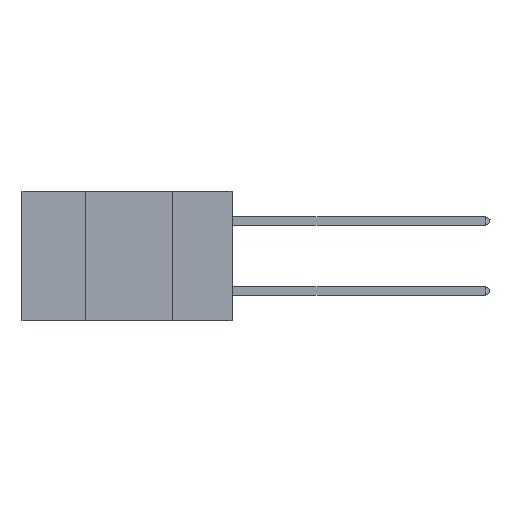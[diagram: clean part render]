
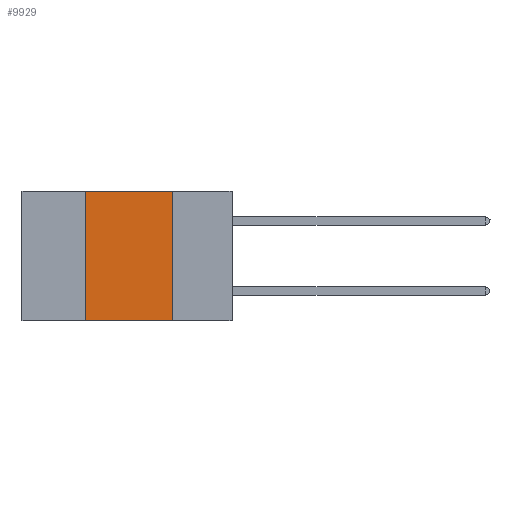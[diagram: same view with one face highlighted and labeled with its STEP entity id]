
A CAD part, left-side view. The second image highlights one B-rep face of the part: STEP entity #9929.
In plain terms, the highlighted planar face has unit normal (-1, 0, 0).
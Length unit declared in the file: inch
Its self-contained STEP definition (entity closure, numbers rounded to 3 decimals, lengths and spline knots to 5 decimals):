
#1337 = ORIENTED_EDGE ( 'NONE', *, *, #12144, .F. ) ;
#2253 = EDGE_CURVE ( 'NONE', #5124, #7362, #2622, .T. ) ;
#2259 = DIRECTION ( 'NONE',  ( 0., 0., 1. ) ) ;
#2405 = FACE_OUTER_BOUND ( 'NONE', #2988, .T. ) ;
#2622 = LINE ( 'NONE', #7259, #3269 ) ;
#2988 = EDGE_LOOP ( 'NONE', ( #16688, #21929, #1337, #7351 ) ) ;
#3269 = VECTOR ( 'NONE', #11135, 39.37008 ) ;
#3982 = CARTESIAN_POINT ( 'NONE',  ( 0., 0.6, -0.37 ) ) ;
#5124 = VERTEX_POINT ( 'NONE', #12665 ) ;
#5948 = VERTEX_POINT ( 'NONE', #15065 ) ;
#7259 = CARTESIAN_POINT ( 'NONE',  ( 0., 0.17, 0. ) ) ;
#7351 = ORIENTED_EDGE ( 'NONE', *, *, #8149, .T. ) ;
#7362 = VERTEX_POINT ( 'NONE', #11038 ) ;
#8149 = EDGE_CURVE ( 'NONE', #5948, #7362, #8484, .T. ) ;
#8484 = LINE ( 'NONE', #3982, #24299 ) ;
#9929 = ADVANCED_FACE ( 'NONE', ( #2405 ), #23775, .F. ) ;
#11038 = CARTESIAN_POINT ( 'NONE',  ( 0., 0.17, -0.37 ) ) ;
#11135 = DIRECTION ( 'NONE',  ( 0., 0., -1. ) ) ;
#11889 = CARTESIAN_POINT ( 'NONE',  ( 0., 0.6, 0. ) ) ;
#12144 = EDGE_CURVE ( 'NONE', #5948, #24886, #24815, .T. ) ;
#12239 = DIRECTION ( 'NONE',  ( 0., -1., 0. ) ) ;
#12665 = CARTESIAN_POINT ( 'NONE',  ( 0., 0.17, 0. ) ) ;
#13498 = VECTOR ( 'NONE', #12239, 39.37008 ) ;
#13648 = VECTOR ( 'NONE', #2259, 39.37008 ) ;
#13874 = DIRECTION ( 'NONE',  ( 0., 0., -1. ) ) ;
#14861 = EDGE_CURVE ( 'NONE', #24886, #5124, #17656, .T. ) ;
#15065 = CARTESIAN_POINT ( 'NONE',  ( 0., 0.42, -0.37 ) ) ;
#16688 = ORIENTED_EDGE ( 'NONE', *, *, #2253, .F. ) ;
#17656 = LINE ( 'NONE', #20222, #13498 ) ;
#17908 = DIRECTION ( 'NONE',  ( 0., -1., 0. ) ) ;
#18241 = CARTESIAN_POINT ( 'NONE',  ( 0., 0.42, 0. ) ) ;
#20222 = CARTESIAN_POINT ( 'NONE',  ( 0., 0.6, 0. ) ) ;
#21483 = CARTESIAN_POINT ( 'NONE',  ( 0., 0.42, 0. ) ) ;
#21929 = ORIENTED_EDGE ( 'NONE', *, *, #14861, .F. ) ;
#23775 = PLANE ( 'NONE',  #25003 ) ;
#24299 = VECTOR ( 'NONE', #17908, 39.37008 ) ;
#24815 = LINE ( 'NONE', #18241, #13648 ) ;
#24886 = VERTEX_POINT ( 'NONE', #21483 ) ;
#25003 = AXIS2_PLACEMENT_3D ( 'NONE', #11889, #25720, #13874 ) ;
#25720 = DIRECTION ( 'NONE',  ( 1., 0., 0. ) ) ;
